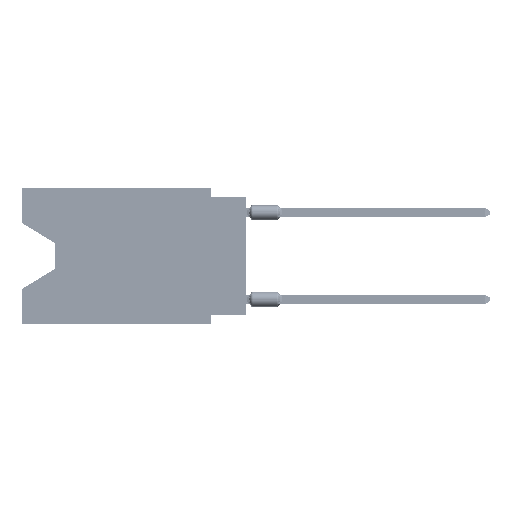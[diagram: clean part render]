
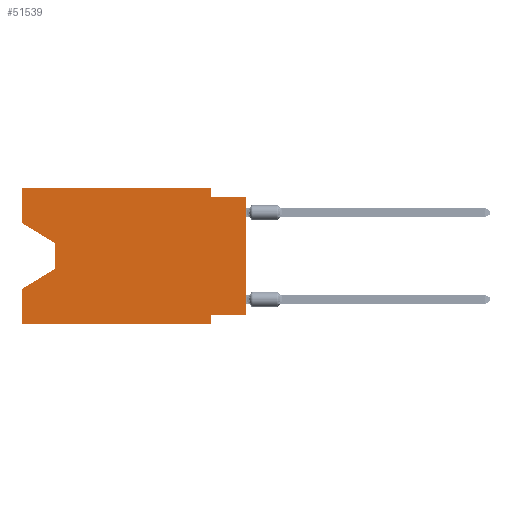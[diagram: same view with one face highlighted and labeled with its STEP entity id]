
A CAD part, left-side view. The second image highlights one B-rep face of the part: STEP entity #51539.
In plain terms, the highlighted planar face has unit normal (-1, 0, 0).
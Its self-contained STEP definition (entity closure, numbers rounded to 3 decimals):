
#125 = CARTESIAN_POINT ( 'NONE',  ( 0., 0., -0.635 ) ) ;
#158 = LINE ( 'NONE', #23179, #64309 ) ;
#926 = ORIENTED_EDGE ( 'NONE', *, *, #65358, .F. ) ;
#1106 = ORIENTED_EDGE ( 'NONE', *, *, #58826, .F. ) ;
#1851 = AXIS2_PLACEMENT_3D ( 'NONE', #34270, #57318, #52026 ) ;
#2106 = VERTEX_POINT ( 'NONE', #49094 ) ;
#2228 = VERTEX_POINT ( 'NONE', #68613 ) ;
#2632 = CARTESIAN_POINT ( 'NONE',  ( 0., 13.97, -5.893 ) ) ;
#3832 = LINE ( 'NONE', #44235, #26638 ) ;
#4387 = DIRECTION ( 'NONE',  ( 0., 0., -1. ) ) ;
#4910 = ORIENTED_EDGE ( 'NONE', *, *, #67573, .F. ) ;
#7293 = CARTESIAN_POINT ( 'NONE',  ( 0., 13.97, -4.013 ) ) ;
#9417 = VERTEX_POINT ( 'NONE', #25960 ) ;
#10426 = DIRECTION ( 'NONE',  ( 0., 0., -1. ) ) ;
#10518 = LINE ( 'NONE', #38818, #33132 ) ;
#10892 = LINE ( 'NONE', #11652, #20764 ) ;
#11091 = CARTESIAN_POINT ( 'NONE',  ( 0., 16.383, -9.906 ) ) ;
#11470 = LINE ( 'NONE', #11091, #22951 ) ;
#11652 = CARTESIAN_POINT ( 'NONE',  ( 0., 16.383, -2.546 ) ) ;
#12369 = VERTEX_POINT ( 'NONE', #21662 ) ;
#12450 = ORIENTED_EDGE ( 'NONE', *, *, #12795, .F. ) ;
#12795 = EDGE_CURVE ( 'NONE', #40083, #9417, #51407, .T. ) ;
#12913 = VERTEX_POINT ( 'NONE', #70274 ) ;
#16022 = CARTESIAN_POINT ( 'NONE',  ( 0., 2.54, -9.906 ) ) ;
#16089 = CARTESIAN_POINT ( 'NONE',  ( 0., 2.54, 0. ) ) ;
#16568 = EDGE_CURVE ( 'NONE', #2228, #63361, #11470, .T. ) ;
#17881 = VERTEX_POINT ( 'NONE', #7293 ) ;
#20764 = VECTOR ( 'NONE', #51664, 1000. ) ;
#21662 = CARTESIAN_POINT ( 'NONE',  ( 0., 2.54, -9.271 ) ) ;
#21807 = ORIENTED_EDGE ( 'NONE', *, *, #23401, .T. ) ;
#22133 = EDGE_CURVE ( 'NONE', #17881, #25601, #56053, .T. ) ;
#22951 = VECTOR ( 'NONE', #45809, 1000. ) ;
#23179 = CARTESIAN_POINT ( 'NONE',  ( 0., 0., 0. ) ) ;
#23401 = EDGE_CURVE ( 'NONE', #12913, #2106, #158, .T. ) ;
#25601 = VERTEX_POINT ( 'NONE', #66205 ) ;
#25960 = CARTESIAN_POINT ( 'NONE',  ( 0., 2.54, 0. ) ) ;
#26638 = VECTOR ( 'NONE', #38566, 1000. ) ;
#27603 = CARTESIAN_POINT ( 'NONE',  ( 0., 16.383, 0. ) ) ;
#27849 = CARTESIAN_POINT ( 'NONE',  ( 0., 16.383, -2.546 ) ) ;
#28317 = CARTESIAN_POINT ( 'NONE',  ( 0., 16.383, -7.36 ) ) ;
#28978 = FACE_OUTER_BOUND ( 'NONE', #44077, .T. ) ;
#33132 = VECTOR ( 'NONE', #50895, 1000. ) ;
#34270 = CARTESIAN_POINT ( 'NONE',  ( 0., 16.383, 0. ) ) ;
#34692 = ORIENTED_EDGE ( 'NONE', *, *, #35207, .T. ) ;
#35207 = EDGE_CURVE ( 'NONE', #25601, #36956, #47955, .T. ) ;
#35951 = EDGE_CURVE ( 'NONE', #12369, #63361, #50825, .T. ) ;
#36956 = VERTEX_POINT ( 'NONE', #28317 ) ;
#38566 = DIRECTION ( 'NONE',  ( 0., 0., 1. ) ) ;
#38818 = CARTESIAN_POINT ( 'NONE',  ( 0., 0., -9.271 ) ) ;
#39034 = CARTESIAN_POINT ( 'NONE',  ( 0., 13.97, -4.013 ) ) ;
#39050 = DIRECTION ( 'NONE',  ( 0., 0., 1. ) ) ;
#39773 = DIRECTION ( 'NONE',  ( 0., -1., 0. ) ) ;
#39961 = EDGE_CURVE ( 'NONE', #51473, #40083, #60497, .T. ) ;
#40083 = VERTEX_POINT ( 'NONE', #63474 ) ;
#42288 = VECTOR ( 'NONE', #39773, 1000. ) ;
#44077 = EDGE_LOOP ( 'NONE', ( #74640, #72802, #34692, #1106, #49663, #55042, #51272, #21807, #4910, #926, #12450, #63663 ) ) ;
#44235 = CARTESIAN_POINT ( 'NONE',  ( 0., 16.383, 0. ) ) ;
#45533 = VERTEX_POINT ( 'NONE', #48541 ) ;
#45809 = DIRECTION ( 'NONE',  ( 0., -1., 0. ) ) ;
#45810 = LINE ( 'NONE', #125, #42288 ) ;
#47657 = CARTESIAN_POINT ( 'NONE',  ( 0., 16.383, 0. ) ) ;
#47955 = LINE ( 'NONE', #2632, #73527 ) ;
#48541 = CARTESIAN_POINT ( 'NONE',  ( 0., 2.54, -0.635 ) ) ;
#49094 = CARTESIAN_POINT ( 'NONE',  ( 0., 0., -0.635 ) ) ;
#49663 = ORIENTED_EDGE ( 'NONE', *, *, #16568, .T. ) ;
#49675 = VECTOR ( 'NONE', #4387, 1000. ) ;
#50282 = DIRECTION ( 'NONE',  ( 0., -1., 0. ) ) ;
#50742 = DIRECTION ( 'NONE',  ( 0., 0., -1. ) ) ;
#50825 = LINE ( 'NONE', #68590, #49675 ) ;
#50895 = DIRECTION ( 'NONE',  ( 0., 1., 0. ) ) ;
#51272 = ORIENTED_EDGE ( 'NONE', *, *, #64909, .F. ) ;
#51407 = LINE ( 'NONE', #27603, #63616 ) ;
#51473 = VERTEX_POINT ( 'NONE', #27849 ) ;
#51539 = ADVANCED_FACE ( 'NONE', ( #28978 ), #73931, .F. ) ;
#51664 = DIRECTION ( 'NONE',  ( 0., -0.855, -0.519 ) ) ;
#52026 = DIRECTION ( 'NONE',  ( 0., 0., -1. ) ) ;
#52894 = DIRECTION ( 'NONE',  ( 0., 0.855, -0.519 ) ) ;
#55042 = ORIENTED_EDGE ( 'NONE', *, *, #35951, .F. ) ;
#56052 = VECTOR ( 'NONE', #50742, 1000. ) ;
#56053 = LINE ( 'NONE', #39034, #56052 ) ;
#56686 = VECTOR ( 'NONE', #10426, 1000. ) ;
#57318 = DIRECTION ( 'NONE',  ( 1., 0., 0. ) ) ;
#58826 = EDGE_CURVE ( 'NONE', #2228, #36956, #3832, .T. ) ;
#58906 = VECTOR ( 'NONE', #65794, 1000. ) ;
#60071 = EDGE_CURVE ( 'NONE', #51473, #17881, #10892, .T. ) ;
#60497 = LINE ( 'NONE', #47657, #58906 ) ;
#63361 = VERTEX_POINT ( 'NONE', #16022 ) ;
#63474 = CARTESIAN_POINT ( 'NONE',  ( 0., 16.383, 0. ) ) ;
#63616 = VECTOR ( 'NONE', #50282, 1000. ) ;
#63663 = ORIENTED_EDGE ( 'NONE', *, *, #39961, .F. ) ;
#64309 = VECTOR ( 'NONE', #39050, 1000. ) ;
#64909 = EDGE_CURVE ( 'NONE', #12913, #12369, #10518, .T. ) ;
#65358 = EDGE_CURVE ( 'NONE', #9417, #45533, #74609, .T. ) ;
#65794 = DIRECTION ( 'NONE',  ( 0., 0., 1. ) ) ;
#66205 = CARTESIAN_POINT ( 'NONE',  ( 0., 13.97, -5.893 ) ) ;
#67573 = EDGE_CURVE ( 'NONE', #45533, #2106, #45810, .T. ) ;
#68590 = CARTESIAN_POINT ( 'NONE',  ( 0., 2.54, -9.906 ) ) ;
#68613 = CARTESIAN_POINT ( 'NONE',  ( 0., 16.383, -9.906 ) ) ;
#70274 = CARTESIAN_POINT ( 'NONE',  ( 0., 0., -9.271 ) ) ;
#72802 = ORIENTED_EDGE ( 'NONE', *, *, #22133, .T. ) ;
#73527 = VECTOR ( 'NONE', #52894, 1000. ) ;
#73931 = PLANE ( 'NONE',  #1851 ) ;
#74609 = LINE ( 'NONE', #16089, #56686 ) ;
#74640 = ORIENTED_EDGE ( 'NONE', *, *, #60071, .T. ) ;
